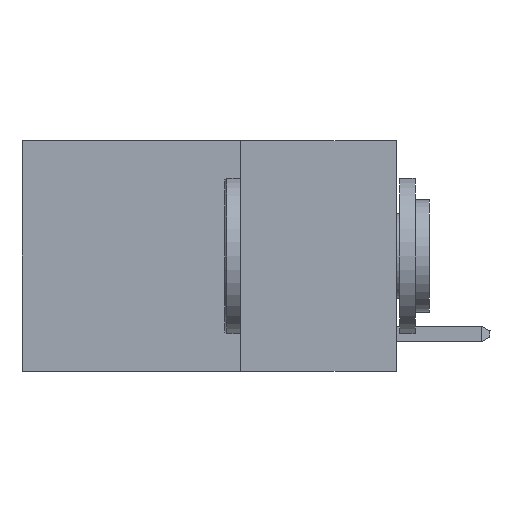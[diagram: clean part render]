
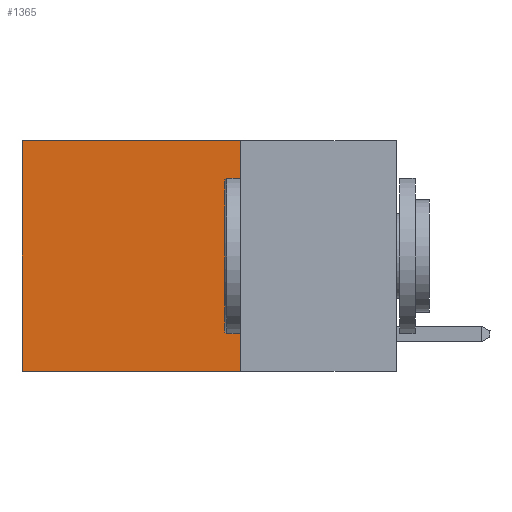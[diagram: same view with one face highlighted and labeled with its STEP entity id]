
A CAD part, left-side view. The second image highlights one B-rep face of the part: STEP entity #1365.
In plain terms, the highlighted planar face has unit normal (-1, 0, 0).
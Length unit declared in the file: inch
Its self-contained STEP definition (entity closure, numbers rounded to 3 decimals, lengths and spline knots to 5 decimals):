
#1365 = ADVANCED_FACE ( 'NONE', ( #8914 ), #24264, .F. ) ;
#1505 = LINE ( 'NONE', #12913, #8206 ) ;
#2581 = VECTOR ( 'NONE', #10677, 39.37008 ) ;
#2910 = CARTESIAN_POINT ( 'NONE',  ( 0.2625, 0.25, -0.37 ) ) ;
#4601 = CARTESIAN_POINT ( 'NONE',  ( 0.2625, 0.6, 0. ) ) ;
#4844 = EDGE_CURVE ( 'NONE', #21558, #20144, #7549, .T. ) ;
#5307 = ORIENTED_EDGE ( 'NONE', *, *, #4844, .T. ) ;
#6815 = ORIENTED_EDGE ( 'NONE', *, *, #22540, .F. ) ;
#6852 = DIRECTION ( 'NONE',  ( 1., 0., 0. ) ) ;
#7549 = LINE ( 'NONE', #16567, #14650 ) ;
#8206 = VECTOR ( 'NONE', #21606, 39.37008 ) ;
#8599 = LINE ( 'NONE', #8750, #2581 ) ;
#8750 = CARTESIAN_POINT ( 'NONE',  ( 0.2625, 0.25, -0.37 ) ) ;
#8914 = FACE_OUTER_BOUND ( 'NONE', #24220, .T. ) ;
#9302 = DIRECTION ( 'NONE',  ( 0., 1., 0. ) ) ;
#10677 = DIRECTION ( 'NONE',  ( 0., 1., 0. ) ) ;
#11263 = VECTOR ( 'NONE', #9302, 39.37008 ) ;
#12913 = CARTESIAN_POINT ( 'NONE',  ( 0.2625, 0.25, 0. ) ) ;
#14650 = VECTOR ( 'NONE', #20853, 39.37008 ) ;
#14836 = CARTESIAN_POINT ( 'NONE',  ( 0.2625, 0.6, -0.37 ) ) ;
#15505 = ORIENTED_EDGE ( 'NONE', *, *, #19039, .T. ) ;
#16567 = CARTESIAN_POINT ( 'NONE',  ( 0.2625, 0.6, 0. ) ) ;
#17239 = CARTESIAN_POINT ( 'NONE',  ( 0.2625, 0.25, 0. ) ) ;
#17932 = DIRECTION ( 'NONE',  ( 0., 0., -1. ) ) ;
#19039 = EDGE_CURVE ( 'NONE', #24536, #21558, #20536, .T. ) ;
#19461 = VERTEX_POINT ( 'NONE', #2910 ) ;
#20144 = VERTEX_POINT ( 'NONE', #14836 ) ;
#20536 = LINE ( 'NONE', #29011, #11263 ) ;
#20853 = DIRECTION ( 'NONE',  ( 0., 0., -1. ) ) ;
#21558 = VERTEX_POINT ( 'NONE', #4601 ) ;
#21606 = DIRECTION ( 'NONE',  ( 0., 0., -1. ) ) ;
#21862 = AXIS2_PLACEMENT_3D ( 'NONE', #22210, #6852, #17932 ) ;
#22210 = CARTESIAN_POINT ( 'NONE',  ( 0.2625, 0.25, 0. ) ) ;
#22540 = EDGE_CURVE ( 'NONE', #19461, #20144, #8599, .T. ) ;
#23216 = ORIENTED_EDGE ( 'NONE', *, *, #23657, .F. ) ;
#23657 = EDGE_CURVE ( 'NONE', #24536, #19461, #1505, .T. ) ;
#24220 = EDGE_LOOP ( 'NONE', ( #5307, #6815, #23216, #15505 ) ) ;
#24264 = PLANE ( 'NONE',  #21862 ) ;
#24536 = VERTEX_POINT ( 'NONE', #17239 ) ;
#29011 = CARTESIAN_POINT ( 'NONE',  ( 0.2625, 0.25, 0. ) ) ;
